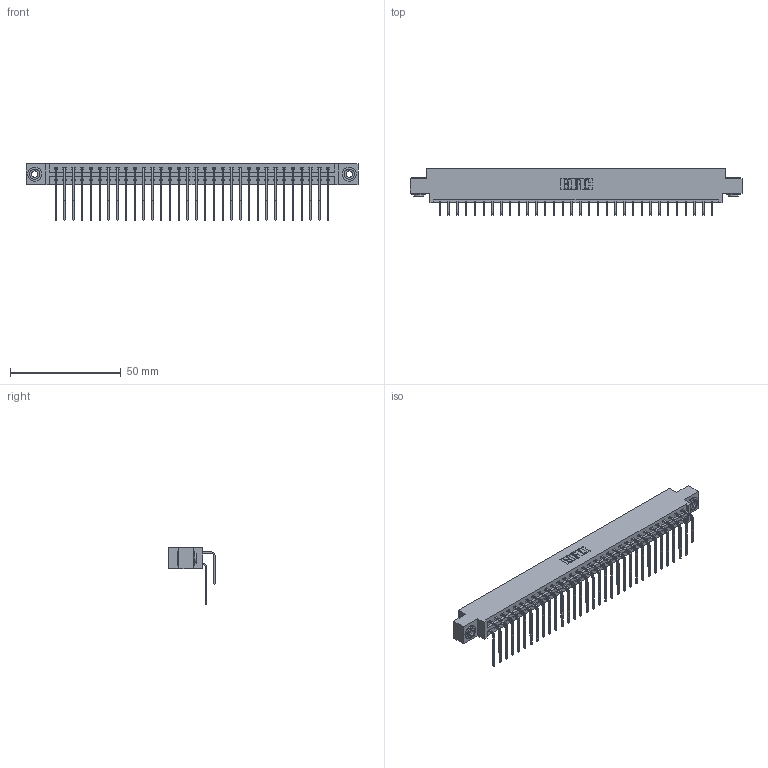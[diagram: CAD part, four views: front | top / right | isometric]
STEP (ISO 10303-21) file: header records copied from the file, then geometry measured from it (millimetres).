
FILE_DESCRIPTION (( 'STEP AP203' ), '1' );
FILE_NAME ('387-064-559-803.STEP', '2019-10-19T17:42:26', ( '' ), ( '' ), 'SwSTEP 2.0', 'SolidWorks 2016', '' );
FILE_SCHEMA (( 'CONFIG_CONTROL_DESIGN' ));
Length unit declared in the file: inch
Products named in the file (5): 345-250-002_345-250-002-102; 345-292-001_559 Tail - 2; 345-292-001_558 559 Tail - 1; 387-064-559-803; 337 Part_0.170 Offset - 0.156 Dia-TH
Assembly tree (67 placements, depth 2):
  387-064-559-803
    337 Part_0.170 Offset - 0.156 Dia-TH
    345-292-001_558 559 Tail - 1  x32
    345-292-001_559 Tail - 2  x32
    345-250-002_345-250-002-102  x2
Bounding box: 149.81 x 20.9 x 25.53 mm (x, y, z)
Volume: 15926.1 mm3; surface area: 20093.4 mm2
Topology: 67 solids, 67 shells, 3740 faces, 11087 edges, 7302 vertices
Faces by surface type: plane 2644, cylinder 1088, cone 8
Entity records: 28670 total; most frequent: CARTESIAN_POINT 4860, ORIENTED_EDGE 4738, DIRECTION 4167, EDGE_CURVE 2369, VECTOR 2177, LINE 2177, VERTEX_POINT 1574, AXIS2_PLACEMENT_3D 995
